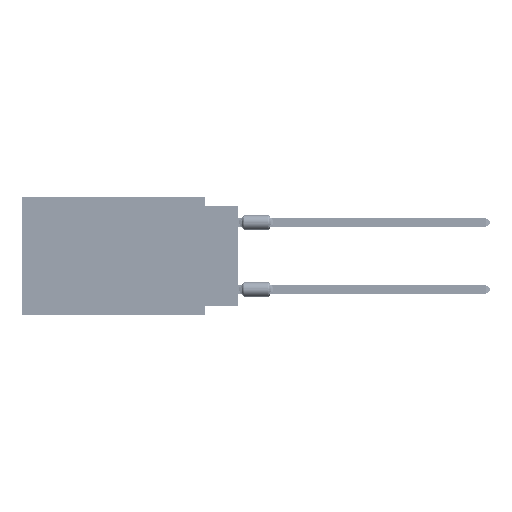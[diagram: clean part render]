
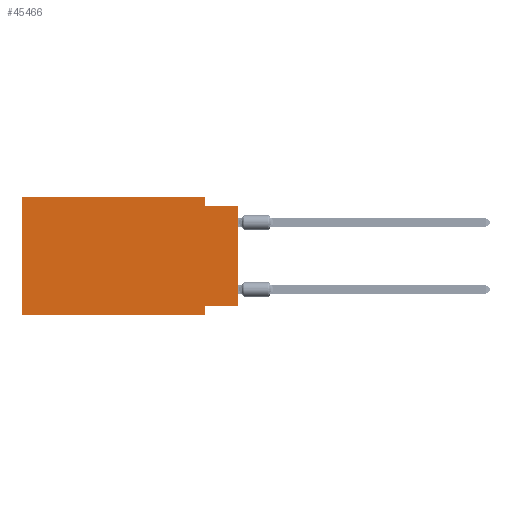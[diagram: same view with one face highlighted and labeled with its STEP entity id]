
A CAD part, left-side view. The second image highlights one B-rep face of the part: STEP entity #45466.
In plain terms, the highlighted planar face has unit normal (-1, 0, 0).
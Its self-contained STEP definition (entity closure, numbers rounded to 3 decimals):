
#100 = DIRECTION ( 'NONE',  ( 0., 0., -1. ) ) ;
#1608 = FACE_OUTER_BOUND ( 'NONE', #48148, .T. ) ;
#6867 = VECTOR ( 'NONE', #100, 1000. ) ;
#7300 = VECTOR ( 'NONE', #15857, 1000. ) ;
#7563 = CARTESIAN_POINT ( 'NONE',  ( 0., 0., -0.635 ) ) ;
#7695 = PLANE ( 'NONE',  #36948 ) ;
#8054 = ORIENTED_EDGE ( 'NONE', *, *, #43658, .T. ) ;
#10324 = ORIENTED_EDGE ( 'NONE', *, *, #63595, .F. ) ;
#10559 = CARTESIAN_POINT ( 'NONE',  ( 0., 0., 0. ) ) ;
#11303 = DIRECTION ( 'NONE',  ( 0., 0., 1. ) ) ;
#12927 = ORIENTED_EDGE ( 'NONE', *, *, #22494, .F. ) ;
#13866 = CARTESIAN_POINT ( 'NONE',  ( 0., 2.54, -0.635 ) ) ;
#14540 = DIRECTION ( 'NONE',  ( 0., 0., -1. ) ) ;
#15857 = DIRECTION ( 'NONE',  ( 0., 0., -1. ) ) ;
#19199 = VERTEX_POINT ( 'NONE', #54814 ) ;
#19837 = EDGE_CURVE ( 'NONE', #30605, #19995, #44801, .T. ) ;
#19995 = VERTEX_POINT ( 'NONE', #13866 ) ;
#21411 = VECTOR ( 'NONE', #49030, 1000. ) ;
#22494 = EDGE_CURVE ( 'NONE', #70174, #49630, #58500, .T. ) ;
#23218 = VERTEX_POINT ( 'NONE', #35725 ) ;
#24274 = CARTESIAN_POINT ( 'NONE',  ( 0., 16.383, -8.89 ) ) ;
#24849 = CARTESIAN_POINT ( 'NONE',  ( 0., 16.383, 0. ) ) ;
#24957 = LINE ( 'NONE', #58889, #43326 ) ;
#25260 = EDGE_CURVE ( 'NONE', #49630, #57501, #58009, .T. ) ;
#26628 = ORIENTED_EDGE ( 'NONE', *, *, #25260, .F. ) ;
#30605 = VERTEX_POINT ( 'NONE', #70990 ) ;
#30894 = ORIENTED_EDGE ( 'NONE', *, *, #62079, .F. ) ;
#33663 = ORIENTED_EDGE ( 'NONE', *, *, #48030, .F. ) ;
#34585 = EDGE_CURVE ( 'NONE', #19199, #57501, #60067, .T. ) ;
#35261 = CARTESIAN_POINT ( 'NONE',  ( 0., 0., -8.255 ) ) ;
#35725 = CARTESIAN_POINT ( 'NONE',  ( 0., 16.383, 0. ) ) ;
#36501 = ORIENTED_EDGE ( 'NONE', *, *, #34585, .T. ) ;
#36948 = AXIS2_PLACEMENT_3D ( 'NONE', #24849, #49215, #14540 ) ;
#37145 = VECTOR ( 'NONE', #65416, 1000. ) ;
#39492 = DIRECTION ( 'NONE',  ( 0., -1., 0. ) ) ;
#40595 = DIRECTION ( 'NONE',  ( 0., 1., 0. ) ) ;
#41855 = CARTESIAN_POINT ( 'NONE',  ( 0., 2.54, -8.89 ) ) ;
#43326 = VECTOR ( 'NONE', #48204, 1000. ) ;
#43658 = EDGE_CURVE ( 'NONE', #70174, #73476, #70000, .T. ) ;
#44328 = VECTOR ( 'NONE', #40595, 1000. ) ;
#44801 = LINE ( 'NONE', #68077, #7300 ) ;
#44836 = LINE ( 'NONE', #68108, #67980 ) ;
#45466 = ADVANCED_FACE ( 'NONE', ( #1608 ), #7695, .F. ) ;
#48030 = EDGE_CURVE ( 'NONE', #19199, #23218, #24957, .T. ) ;
#48148 = EDGE_LOOP ( 'NONE', ( #8054, #10324, #72342, #30894, #33663, #36501, #26628, #12927 ) ) ;
#48204 = DIRECTION ( 'NONE',  ( 0., 0., 1. ) ) ;
#48266 = CARTESIAN_POINT ( 'NONE',  ( 0., 2.54, -8.255 ) ) ;
#49030 = DIRECTION ( 'NONE',  ( 0., -1., 0. ) ) ;
#49215 = DIRECTION ( 'NONE',  ( 1., 0., 0. ) ) ;
#49630 = VERTEX_POINT ( 'NONE', #48266 ) ;
#52295 = CARTESIAN_POINT ( 'NONE',  ( 0., 2.54, -8.89 ) ) ;
#53554 = CARTESIAN_POINT ( 'NONE',  ( 0., 0., -8.255 ) ) ;
#54374 = LINE ( 'NONE', #72293, #21411 ) ;
#54814 = CARTESIAN_POINT ( 'NONE',  ( 0., 16.383, -8.89 ) ) ;
#57501 = VERTEX_POINT ( 'NONE', #41855 ) ;
#58009 = LINE ( 'NONE', #52295, #6867 ) ;
#58500 = LINE ( 'NONE', #35261, #44328 ) ;
#58889 = CARTESIAN_POINT ( 'NONE',  ( 0., 16.383, 0. ) ) ;
#60067 = LINE ( 'NONE', #24274, #37145 ) ;
#62079 = EDGE_CURVE ( 'NONE', #23218, #30605, #54374, .T. ) ;
#63595 = EDGE_CURVE ( 'NONE', #19995, #73476, #44836, .T. ) ;
#65416 = DIRECTION ( 'NONE',  ( 0., -1., 0. ) ) ;
#66934 = VECTOR ( 'NONE', #11303, 1000. ) ;
#67980 = VECTOR ( 'NONE', #39492, 1000. ) ;
#68077 = CARTESIAN_POINT ( 'NONE',  ( 0., 2.54, 0. ) ) ;
#68108 = CARTESIAN_POINT ( 'NONE',  ( 0., 0., -0.635 ) ) ;
#70000 = LINE ( 'NONE', #10559, #66934 ) ;
#70174 = VERTEX_POINT ( 'NONE', #53554 ) ;
#70990 = CARTESIAN_POINT ( 'NONE',  ( 0., 2.54, 0. ) ) ;
#72293 = CARTESIAN_POINT ( 'NONE',  ( 0., 16.383, 0. ) ) ;
#72342 = ORIENTED_EDGE ( 'NONE', *, *, #19837, .F. ) ;
#73476 = VERTEX_POINT ( 'NONE', #7563 ) ;
